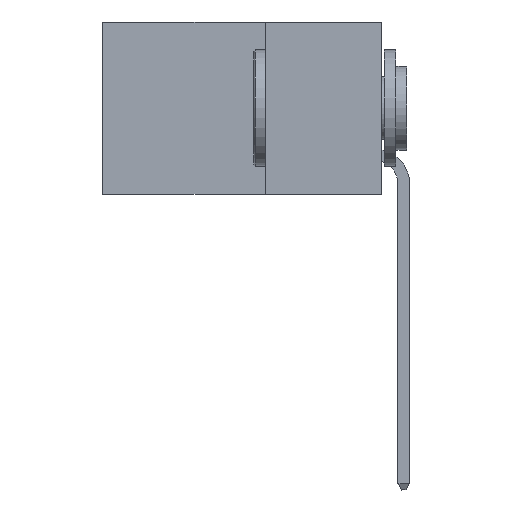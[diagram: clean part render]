
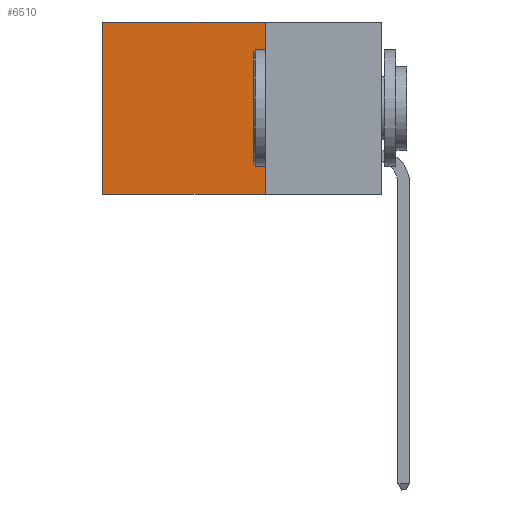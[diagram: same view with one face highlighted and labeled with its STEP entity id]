
A CAD part, left-side view. The second image highlights one B-rep face of the part: STEP entity #6510.
In plain terms, the highlighted planar face has unit normal (-1, 0, 0).
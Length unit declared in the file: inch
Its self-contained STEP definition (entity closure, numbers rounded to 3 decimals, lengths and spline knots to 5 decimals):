
#51 = CARTESIAN_POINT ( 'NONE',  ( 0.2875, 0.25, 0. ) ) ;
#562 = CARTESIAN_POINT ( 'NONE',  ( 0.2875, 0.25, 0. ) ) ;
#2000 = VECTOR ( 'NONE', #9304, 39.37008 ) ;
#2025 = LINE ( 'NONE', #6739, #16035 ) ;
#2042 = ORIENTED_EDGE ( 'NONE', *, *, #17865, .T. ) ;
#4365 = VERTEX_POINT ( 'NONE', #18715 ) ;
#4438 = LINE ( 'NONE', #51, #18208 ) ;
#5112 = DIRECTION ( 'NONE',  ( 1., 0., 0. ) ) ;
#6209 = VERTEX_POINT ( 'NONE', #10302 ) ;
#6510 = ADVANCED_FACE ( 'NONE', ( #17240 ), #6524, .F. ) ;
#6524 = PLANE ( 'NONE',  #8520 ) ;
#6739 = CARTESIAN_POINT ( 'NONE',  ( 0.2875, 0.25, -0.37 ) ) ;
#6759 = CARTESIAN_POINT ( 'NONE',  ( 0.2875, 0.6, -0.37 ) ) ;
#7189 = LINE ( 'NONE', #13889, #10696 ) ;
#7607 = CARTESIAN_POINT ( 'NONE',  ( 0.2875, 0.25, -0.37 ) ) ;
#8520 = AXIS2_PLACEMENT_3D ( 'NONE', #562, #5112, #18555 ) ;
#9188 = ORIENTED_EDGE ( 'NONE', *, *, #18167, .F. ) ;
#9304 = DIRECTION ( 'NONE',  ( 0., 0., -1. ) ) ;
#9365 = ORIENTED_EDGE ( 'NONE', *, *, #14900, .T. ) ;
#9923 = LINE ( 'NONE', #18203, #2000 ) ;
#10302 = CARTESIAN_POINT ( 'NONE',  ( 0.2875, 0.6, 0. ) ) ;
#10515 = DIRECTION ( 'NONE',  ( 0., 1., 0. ) ) ;
#10696 = VECTOR ( 'NONE', #13824, 39.37008 ) ;
#11189 = DIRECTION ( 'NONE',  ( 0., 1., 0. ) ) ;
#13824 = DIRECTION ( 'NONE',  ( 0., 0., -1. ) ) ;
#13889 = CARTESIAN_POINT ( 'NONE',  ( 0.2875, 0.25, 0. ) ) ;
#14900 = EDGE_CURVE ( 'NONE', #4365, #6209, #4438, .T. ) ;
#15194 = EDGE_CURVE ( 'NONE', #4365, #16551, #7189, .T. ) ;
#16035 = VECTOR ( 'NONE', #11189, 39.37008 ) ;
#16036 = EDGE_LOOP ( 'NONE', ( #2042, #9188, #17077, #9365 ) ) ;
#16551 = VERTEX_POINT ( 'NONE', #7607 ) ;
#17077 = ORIENTED_EDGE ( 'NONE', *, *, #15194, .F. ) ;
#17240 = FACE_OUTER_BOUND ( 'NONE', #16036, .T. ) ;
#17411 = VERTEX_POINT ( 'NONE', #6759 ) ;
#17865 = EDGE_CURVE ( 'NONE', #6209, #17411, #9923, .T. ) ;
#18167 = EDGE_CURVE ( 'NONE', #16551, #17411, #2025, .T. ) ;
#18203 = CARTESIAN_POINT ( 'NONE',  ( 0.2875, 0.6, 0. ) ) ;
#18208 = VECTOR ( 'NONE', #10515, 39.37008 ) ;
#18555 = DIRECTION ( 'NONE',  ( 0., 0., -1. ) ) ;
#18715 = CARTESIAN_POINT ( 'NONE',  ( 0.2875, 0.25, 0. ) ) ;
